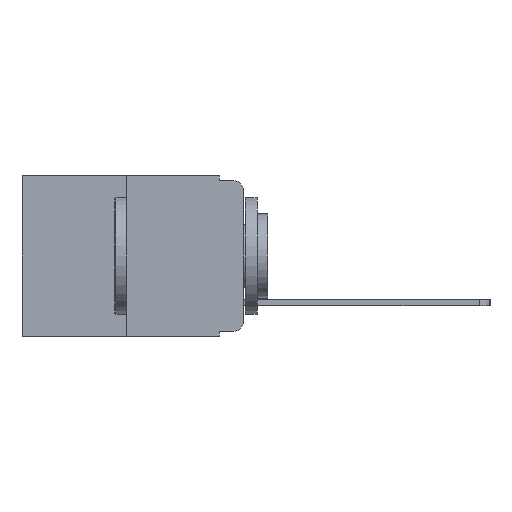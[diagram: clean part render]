
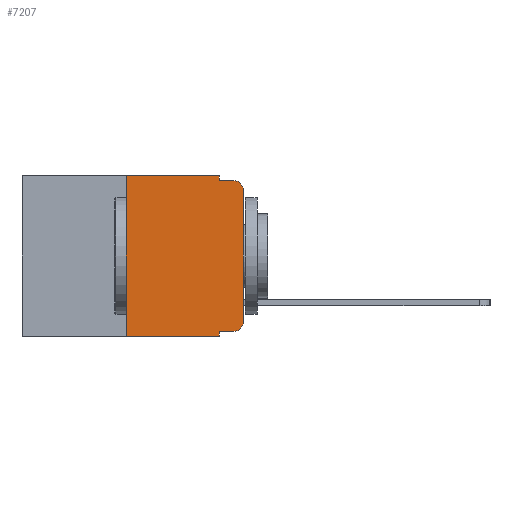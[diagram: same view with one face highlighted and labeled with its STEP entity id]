
A CAD part, left-side view. The second image highlights one B-rep face of the part: STEP entity #7207.
In plain terms, the highlighted planar face has unit normal (-1, 0, 0).
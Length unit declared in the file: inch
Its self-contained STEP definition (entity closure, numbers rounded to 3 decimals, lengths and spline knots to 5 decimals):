
#176 = ORIENTED_EDGE ( 'NONE', *, *, #8027, .F. ) ;
#363 = AXIS2_PLACEMENT_3D ( 'NONE', #12213, #6788, #801 ) ;
#414 = CIRCLE ( 'NONE', #7178, 0.02 ) ;
#471 = LINE ( 'NONE', #6853, #10201 ) ;
#475 = DIRECTION ( 'NONE',  ( 0., -1., 0. ) ) ;
#657 = VECTOR ( 'NONE', #11002, 39.37008 ) ;
#703 = CARTESIAN_POINT ( 'NONE',  ( 0., 0.051, -0.333 ) ) ;
#801 = DIRECTION ( 'NONE',  ( 0., 0., -1. ) ) ;
#1267 = EDGE_CURVE ( 'NONE', #11833, #4041, #10341, .T. ) ;
#1419 = LINE ( 'NONE', #3698, #11272 ) ;
#1974 = EDGE_CURVE ( 'NONE', #4252, #2228, #471, .T. ) ;
#2228 = VERTEX_POINT ( 'NONE', #4351 ) ;
#2426 = VERTEX_POINT ( 'NONE', #7975 ) ;
#2442 = FACE_OUTER_BOUND ( 'NONE', #4053, .T. ) ;
#2629 = ORIENTED_EDGE ( 'NONE', *, *, #12326, .F. ) ;
#2639 = CARTESIAN_POINT ( 'NONE',  ( 0., 0., 0. ) ) ;
#2716 = CARTESIAN_POINT ( 'NONE',  ( 0., 0.02, -0.333 ) ) ;
#2951 = VERTEX_POINT ( 'NONE', #9161 ) ;
#3238 = CARTESIAN_POINT ( 'NONE',  ( 0., 0.473, 0. ) ) ;
#3303 = ORIENTED_EDGE ( 'NONE', *, *, #1974, .F. ) ;
#3380 = EDGE_CURVE ( 'NONE', #11833, #4545, #1419, .T. ) ;
#3426 = CIRCLE ( 'NONE', #363, 0.02 ) ;
#3526 = CARTESIAN_POINT ( 'NONE',  ( 0., 0., -0.03 ) ) ;
#3621 = ORIENTED_EDGE ( 'NONE', *, *, #1267, .F. ) ;
#3698 = CARTESIAN_POINT ( 'NONE',  ( 0., 0.051, -0.333 ) ) ;
#3839 = VERTEX_POINT ( 'NONE', #11389 ) ;
#4015 = EDGE_CURVE ( 'NONE', #4545, #2951, #414, .T. ) ;
#4041 = VERTEX_POINT ( 'NONE', #11268 ) ;
#4053 = EDGE_LOOP ( 'NONE', ( #4977, #7514, #2629, #7820, #176, #3303, #8390, #3621, #11060, #8942 ) ) ;
#4112 = PLANE ( 'NONE',  #6032 ) ;
#4252 = VERTEX_POINT ( 'NONE', #9406 ) ;
#4351 = CARTESIAN_POINT ( 'NONE',  ( 0., 0.25, 0. ) ) ;
#4480 = DIRECTION ( 'NONE',  ( 0., -1., 0. ) ) ;
#4545 = VERTEX_POINT ( 'NONE', #2716 ) ;
#4977 = ORIENTED_EDGE ( 'NONE', *, *, #11123, .T. ) ;
#5109 = CARTESIAN_POINT ( 'NONE',  ( 0., 0.473, 0. ) ) ;
#5157 = VECTOR ( 'NONE', #8043, 39.37008 ) ;
#5518 = CARTESIAN_POINT ( 'NONE',  ( 0., 0.051, 0. ) ) ;
#5822 = EDGE_CURVE ( 'NONE', #4252, #4041, #11069, .T. ) ;
#6032 = AXIS2_PLACEMENT_3D ( 'NONE', #5109, #11542, #6086 ) ;
#6086 = DIRECTION ( 'NONE',  ( 0., 0., -1. ) ) ;
#6218 = VECTOR ( 'NONE', #10899, 39.37008 ) ;
#6254 = CARTESIAN_POINT ( 'NONE',  ( 0., 0.02, -0.01 ) ) ;
#6350 = CARTESIAN_POINT ( 'NONE',  ( 0., 0.473, -0.343 ) ) ;
#6424 = VERTEX_POINT ( 'NONE', #6254 ) ;
#6788 = DIRECTION ( 'NONE',  ( -1., 0., 0. ) ) ;
#6853 = CARTESIAN_POINT ( 'NONE',  ( 0., 0.25, 0. ) ) ;
#7003 = DIRECTION ( 'NONE',  ( 0., 0., 1. ) ) ;
#7178 = AXIS2_PLACEMENT_3D ( 'NONE', #12206, #12204, #11143 ) ;
#7207 = ADVANCED_FACE ( 'NONE', ( #2442 ), #4112, .F. ) ;
#7382 = LINE ( 'NONE', #3238, #5157 ) ;
#7514 = ORIENTED_EDGE ( 'NONE', *, *, #9941, .T. ) ;
#7820 = ORIENTED_EDGE ( 'NONE', *, *, #11716, .F. ) ;
#7975 = CARTESIAN_POINT ( 'NONE',  ( 0., 0.051, -0.01 ) ) ;
#8027 = EDGE_CURVE ( 'NONE', #2228, #3839, #7382, .T. ) ;
#8043 = DIRECTION ( 'NONE',  ( 0., -1., 0. ) ) ;
#8390 = ORIENTED_EDGE ( 'NONE', *, *, #5822, .T. ) ;
#8503 = LINE ( 'NONE', #5518, #657 ) ;
#8942 = ORIENTED_EDGE ( 'NONE', *, *, #4015, .T. ) ;
#9161 = CARTESIAN_POINT ( 'NONE',  ( 0., 0., -0.313 ) ) ;
#9187 = CARTESIAN_POINT ( 'NONE',  ( 0., 0.051, -0.01 ) ) ;
#9201 = VECTOR ( 'NONE', #4480, 39.37008 ) ;
#9339 = DIRECTION ( 'NONE',  ( 0., 0., 1. ) ) ;
#9406 = CARTESIAN_POINT ( 'NONE',  ( 0., 0.25, -0.343 ) ) ;
#9854 = DIRECTION ( 'NONE',  ( 0., 0., -1. ) ) ;
#9941 = EDGE_CURVE ( 'NONE', #12317, #6424, #3426, .T. ) ;
#9995 = CARTESIAN_POINT ( 'NONE',  ( 0., 0.051, 0. ) ) ;
#10058 = VECTOR ( 'NONE', #9854, 39.37008 ) ;
#10201 = VECTOR ( 'NONE', #7003, 39.37008 ) ;
#10341 = LINE ( 'NONE', #9995, #10058 ) ;
#10899 = DIRECTION ( 'NONE',  ( 0., -1., 0. ) ) ;
#11002 = DIRECTION ( 'NONE',  ( 0., 0., -1. ) ) ;
#11060 = ORIENTED_EDGE ( 'NONE', *, *, #3380, .T. ) ;
#11069 = LINE ( 'NONE', #6350, #6218 ) ;
#11123 = EDGE_CURVE ( 'NONE', #2951, #12317, #12030, .T. ) ;
#11143 = DIRECTION ( 'NONE',  ( 0., 0., -1. ) ) ;
#11268 = CARTESIAN_POINT ( 'NONE',  ( 0., 0.051, -0.343 ) ) ;
#11272 = VECTOR ( 'NONE', #475, 39.37008 ) ;
#11389 = CARTESIAN_POINT ( 'NONE',  ( 0., 0.051, 0. ) ) ;
#11542 = DIRECTION ( 'NONE',  ( 1., 0., 0. ) ) ;
#11577 = LINE ( 'NONE', #9187, #9201 ) ;
#11716 = EDGE_CURVE ( 'NONE', #3839, #2426, #8503, .T. ) ;
#11833 = VERTEX_POINT ( 'NONE', #703 ) ;
#12030 = LINE ( 'NONE', #2639, #12310 ) ;
#12204 = DIRECTION ( 'NONE',  ( -1., 0., 0. ) ) ;
#12206 = CARTESIAN_POINT ( 'NONE',  ( 0., 0.02, -0.313 ) ) ;
#12213 = CARTESIAN_POINT ( 'NONE',  ( 0., 0.02, -0.03 ) ) ;
#12310 = VECTOR ( 'NONE', #9339, 39.37008 ) ;
#12317 = VERTEX_POINT ( 'NONE', #3526 ) ;
#12326 = EDGE_CURVE ( 'NONE', #2426, #6424, #11577, .T. ) ;
